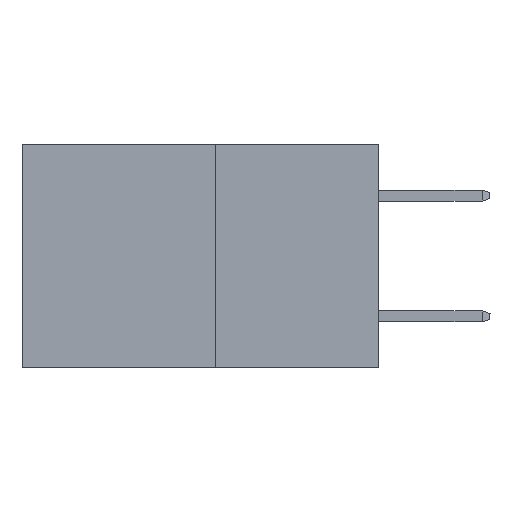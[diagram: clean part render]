
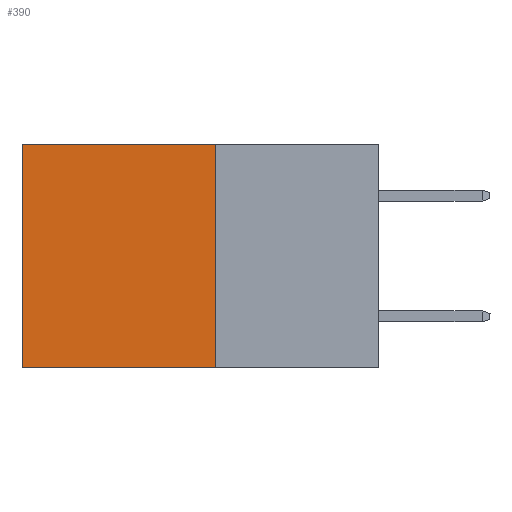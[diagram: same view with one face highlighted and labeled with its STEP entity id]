
A CAD part, left-side view. The second image highlights one B-rep face of the part: STEP entity #390.
In plain terms, the highlighted planar face has unit normal (-1, 0, 0).
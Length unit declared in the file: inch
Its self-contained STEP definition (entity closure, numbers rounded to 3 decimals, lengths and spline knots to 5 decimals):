
#390 = ADVANCED_FACE ( 'NONE', ( #21613 ), #6032, .F. ) ;
#400 = EDGE_CURVE ( 'NONE', #10536, #4638, #5515, .T. ) ;
#571 = VECTOR ( 'NONE', #2750, 39.37008 ) ;
#2416 = VERTEX_POINT ( 'NONE', #2951 ) ;
#2533 = ORIENTED_EDGE ( 'NONE', *, *, #13437, .T. ) ;
#2750 = DIRECTION ( 'NONE',  ( 0., 0., -1. ) ) ;
#2951 = CARTESIAN_POINT ( 'NONE',  ( 0.277, 0.59, 0. ) ) ;
#3216 = CARTESIAN_POINT ( 'NONE',  ( 0.277, 0.27, -0.37 ) ) ;
#4555 = VECTOR ( 'NONE', #6127, 39.37008 ) ;
#4638 = VERTEX_POINT ( 'NONE', #16722 ) ;
#5515 = LINE ( 'NONE', #3216, #571 ) ;
#5828 = CARTESIAN_POINT ( 'NONE',  ( 0.277, 0.27, -0.37 ) ) ;
#5895 = EDGE_CURVE ( 'NONE', #10536, #2416, #10206, .T. ) ;
#6032 = PLANE ( 'NONE',  #15685 ) ;
#6127 = DIRECTION ( 'NONE',  ( 0., 1., 0. ) ) ;
#6804 = ORIENTED_EDGE ( 'NONE', *, *, #400, .F. ) ;
#7109 = CARTESIAN_POINT ( 'NONE',  ( 0.277, 0.27, 0. ) ) ;
#7146 = ORIENTED_EDGE ( 'NONE', *, *, #16538, .F. ) ;
#9075 = CARTESIAN_POINT ( 'NONE',  ( 0.277, 0.59, -0.37 ) ) ;
#10187 = LINE ( 'NONE', #22333, #26833 ) ;
#10206 = LINE ( 'NONE', #26991, #4555 ) ;
#10536 = VERTEX_POINT ( 'NONE', #7109 ) ;
#11356 = ORIENTED_EDGE ( 'NONE', *, *, #5895, .T. ) ;
#11431 = CARTESIAN_POINT ( 'NONE',  ( 0.277, 0.27, -0.37 ) ) ;
#13437 = EDGE_CURVE ( 'NONE', #2416, #16480, #10187, .T. ) ;
#15000 = DIRECTION ( 'NONE',  ( 1., 0., 0. ) ) ;
#15685 = AXIS2_PLACEMENT_3D ( 'NONE', #5828, #15000, #26806 ) ;
#15779 = VECTOR ( 'NONE', #23920, 39.37008 ) ;
#16480 = VERTEX_POINT ( 'NONE', #9075 ) ;
#16538 = EDGE_CURVE ( 'NONE', #4638, #16480, #17109, .T. ) ;
#16722 = CARTESIAN_POINT ( 'NONE',  ( 0.277, 0.27, -0.37 ) ) ;
#17109 = LINE ( 'NONE', #11431, #15779 ) ;
#21613 = FACE_OUTER_BOUND ( 'NONE', #22818, .T. ) ;
#22333 = CARTESIAN_POINT ( 'NONE',  ( 0.277, 0.59, -0.37 ) ) ;
#22818 = EDGE_LOOP ( 'NONE', ( #2533, #7146, #6804, #11356 ) ) ;
#23920 = DIRECTION ( 'NONE',  ( 0., 1., 0. ) ) ;
#26493 = DIRECTION ( 'NONE',  ( 0., 0., -1. ) ) ;
#26806 = DIRECTION ( 'NONE',  ( 0., 0., -1. ) ) ;
#26833 = VECTOR ( 'NONE', #26493, 39.37008 ) ;
#26991 = CARTESIAN_POINT ( 'NONE',  ( 0.277, 0.27, 0. ) ) ;
